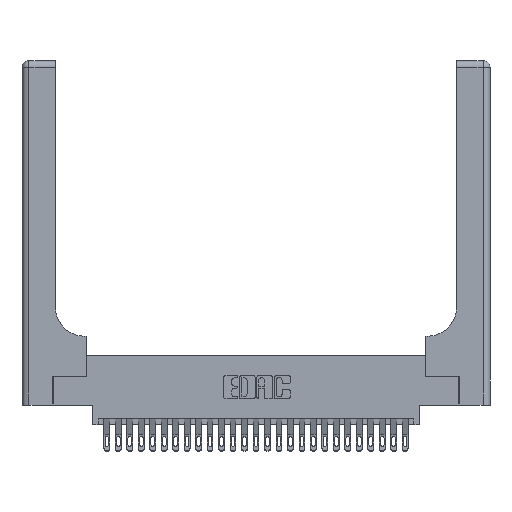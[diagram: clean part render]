
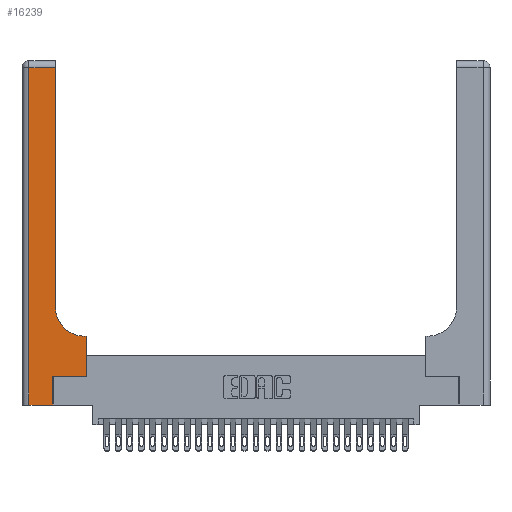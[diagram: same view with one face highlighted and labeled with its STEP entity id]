
A CAD part, top view. The second image highlights one B-rep face of the part: STEP entity #16239.
In plain terms, the highlighted planar face has unit normal (0, 0, 1).
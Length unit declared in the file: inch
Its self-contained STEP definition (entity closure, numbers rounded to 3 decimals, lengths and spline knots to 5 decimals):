
#832 = VERTEX_POINT ( 'NONE', #2992 ) ;
#997 = ORIENTED_EDGE ( 'NONE', *, *, #23672, .T. ) ;
#1411 = VECTOR ( 'NONE', #24004, 39.37008 ) ;
#1450 = VERTEX_POINT ( 'NONE', #12445 ) ;
#1514 = EDGE_LOOP ( 'NONE', ( #9467, #15440, #22699, #5614, #11589, #18245, #997, #13708, #25479 ) ) ;
#1756 = EDGE_CURVE ( 'NONE', #4194, #26156, #10470, .T. ) ;
#1829 = CARTESIAN_POINT ( 'NONE',  ( 0.06, 0., 0.37 ) ) ;
#2924 = LINE ( 'NONE', #6574, #14209 ) ;
#2992 = CARTESIAN_POINT ( 'NONE',  ( 0.5585, 0.6, 0.37 ) ) ;
#3106 = CARTESIAN_POINT ( 'NONE',  ( 0., 3., 0.37 ) ) ;
#4124 = CARTESIAN_POINT ( 'NONE',  ( 0.5415, 0.85, 0.37 ) ) ;
#4140 = CARTESIAN_POINT ( 'NONE',  ( 0.2915, 3., 0.37 ) ) ;
#4194 = VERTEX_POINT ( 'NONE', #1829 ) ;
#4478 = VECTOR ( 'NONE', #8831, 39.37008 ) ;
#4530 = VECTOR ( 'NONE', #28844, 39.37008 ) ;
#5614 = ORIENTED_EDGE ( 'NONE', *, *, #1756, .T. ) ;
#6162 = CARTESIAN_POINT ( 'NONE',  ( 0.06, 3., 0.37 ) ) ;
#6380 = DIRECTION ( 'NONE',  ( 1., 0., 0. ) ) ;
#6393 = DIRECTION ( 'NONE',  ( 0., 1., 0. ) ) ;
#6569 = VECTOR ( 'NONE', #6393, 39.37008 ) ;
#6574 = CARTESIAN_POINT ( 'NONE',  ( 0.2915, 0.6, 0.37 ) ) ;
#7479 = EDGE_CURVE ( 'NONE', #23393, #1450, #20601, .T. ) ;
#7667 = DIRECTION ( 'NONE',  ( -1., 0., 0. ) ) ;
#7824 = CARTESIAN_POINT ( 'NONE',  ( 0.5585, 0.25, 0.37 ) ) ;
#8143 = CARTESIAN_POINT ( 'NONE',  ( 0.269, 0., 0.37 ) ) ;
#8831 = DIRECTION ( 'NONE',  ( 0., 1., 0. ) ) ;
#8944 = VERTEX_POINT ( 'NONE', #23197 ) ;
#9378 = CARTESIAN_POINT ( 'NONE',  ( 0.2915, 0.85, 0.37 ) ) ;
#9467 = ORIENTED_EDGE ( 'NONE', *, *, #23586, .T. ) ;
#10063 = VECTOR ( 'NONE', #12741, 39.37008 ) ;
#10469 = EDGE_CURVE ( 'NONE', #1450, #4194, #12698, .T. ) ;
#10470 = LINE ( 'NONE', #13433, #4530 ) ;
#10540 = CARTESIAN_POINT ( 'NONE',  ( 0.269, 0., 0.37 ) ) ;
#11589 = ORIENTED_EDGE ( 'NONE', *, *, #27168, .T. ) ;
#12445 = CARTESIAN_POINT ( 'NONE',  ( 0.06, 2.94, 0.37 ) ) ;
#12698 = LINE ( 'NONE', #6162, #1411 ) ;
#12741 = DIRECTION ( 'NONE',  ( 1., 0., 0. ) ) ;
#13433 = CARTESIAN_POINT ( 'NONE',  ( 0., 0., 0.37 ) ) ;
#13600 = CARTESIAN_POINT ( 'NONE',  ( 0., 2.94, 0.37 ) ) ;
#13639 = EDGE_CURVE ( 'NONE', #17896, #21194, #27065, .T. ) ;
#13708 = ORIENTED_EDGE ( 'NONE', *, *, #18496, .T. ) ;
#14209 = VECTOR ( 'NONE', #22249, 39.37008 ) ;
#15009 = CARTESIAN_POINT ( 'NONE',  ( 0.269, 0.25, 0.37 ) ) ;
#15440 = ORIENTED_EDGE ( 'NONE', *, *, #7479, .T. ) ;
#15512 = AXIS2_PLACEMENT_3D ( 'NONE', #4124, #19781, #6380 ) ;
#16153 = LINE ( 'NONE', #10540, #21356 ) ;
#16239 = ADVANCED_FACE ( 'NONE', ( #22936 ), #16572, .F. ) ;
#16572 = PLANE ( 'NONE',  #22470 ) ;
#17896 = VERTEX_POINT ( 'NONE', #22369 ) ;
#18088 = DIRECTION ( 'NONE',  ( -1., 0., 0. ) ) ;
#18245 = ORIENTED_EDGE ( 'NONE', *, *, #13639, .T. ) ;
#18496 = EDGE_CURVE ( 'NONE', #832, #8944, #2924, .T. ) ;
#18916 = EDGE_CURVE ( 'NONE', #8944, #28607, #21461, .T. ) ;
#19781 = DIRECTION ( 'NONE',  ( 0., 0., -1. ) ) ;
#19921 = VECTOR ( 'NONE', #18088, 39.37008 ) ;
#19980 = CARTESIAN_POINT ( 'NONE',  ( 0.5585, 0.25, 0.37 ) ) ;
#20601 = LINE ( 'NONE', #13600, #19921 ) ;
#21036 = DIRECTION ( 'NONE',  ( 0., 0., -1. ) ) ;
#21194 = VERTEX_POINT ( 'NONE', #7824 ) ;
#21356 = VECTOR ( 'NONE', #23857, 39.37008 ) ;
#21461 = CIRCLE ( 'NONE', #15512, 0.25 ) ;
#22245 = LINE ( 'NONE', #19980, #4478 ) ;
#22249 = DIRECTION ( 'NONE',  ( -1., 0., 0. ) ) ;
#22369 = CARTESIAN_POINT ( 'NONE',  ( 0.269, 0.25, 0.37 ) ) ;
#22470 = AXIS2_PLACEMENT_3D ( 'NONE', #3106, #21036, #7667 ) ;
#22699 = ORIENTED_EDGE ( 'NONE', *, *, #10469, .T. ) ;
#22936 = FACE_OUTER_BOUND ( 'NONE', #1514, .T. ) ;
#23197 = CARTESIAN_POINT ( 'NONE',  ( 0.5415, 0.6, 0.37 ) ) ;
#23393 = VERTEX_POINT ( 'NONE', #25751 ) ;
#23586 = EDGE_CURVE ( 'NONE', #28607, #23393, #24357, .T. ) ;
#23672 = EDGE_CURVE ( 'NONE', #21194, #832, #22245, .T. ) ;
#23857 = DIRECTION ( 'NONE',  ( 0., 1., 0. ) ) ;
#24004 = DIRECTION ( 'NONE',  ( 0., -1., 0. ) ) ;
#24357 = LINE ( 'NONE', #4140, #6569 ) ;
#25479 = ORIENTED_EDGE ( 'NONE', *, *, #18916, .T. ) ;
#25751 = CARTESIAN_POINT ( 'NONE',  ( 0.2915, 2.94, 0.37 ) ) ;
#26156 = VERTEX_POINT ( 'NONE', #8143 ) ;
#27065 = LINE ( 'NONE', #15009, #10063 ) ;
#27168 = EDGE_CURVE ( 'NONE', #26156, #17896, #16153, .T. ) ;
#28607 = VERTEX_POINT ( 'NONE', #9378 ) ;
#28844 = DIRECTION ( 'NONE',  ( 1., 0., 0. ) ) ;
